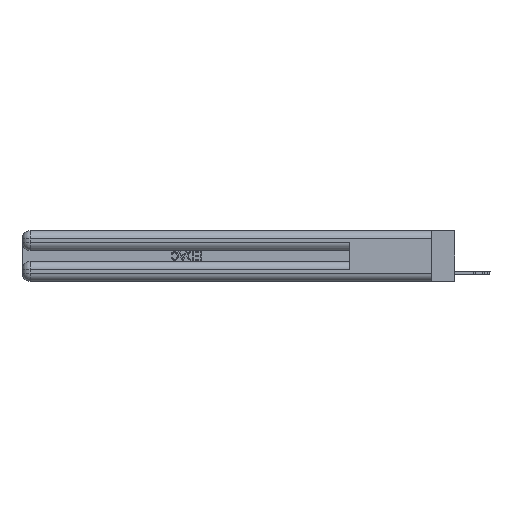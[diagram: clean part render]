
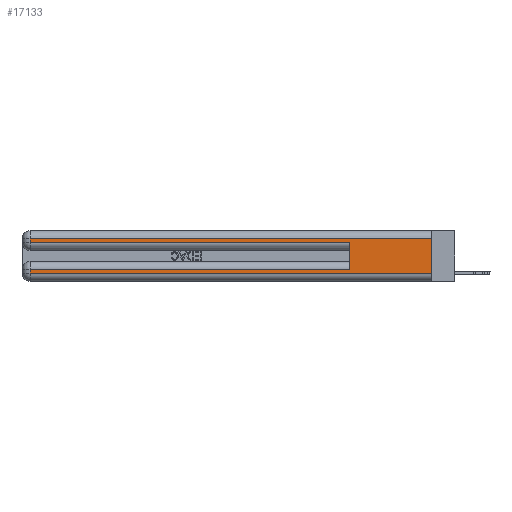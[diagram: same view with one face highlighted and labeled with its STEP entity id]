
A CAD part, left-side view. The second image highlights one B-rep face of the part: STEP entity #17133.
In plain terms, the highlighted planar face has unit normal (-1, 0, 0).
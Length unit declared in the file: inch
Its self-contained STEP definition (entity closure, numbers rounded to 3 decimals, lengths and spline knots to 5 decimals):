
#374 = CARTESIAN_POINT ( 'NONE',  ( 0., 0., 0.06 ) ) ;
#433 = FACE_OUTER_BOUND ( 'NONE', #507, .T. ) ;
#507 = EDGE_LOOP ( 'NONE', ( #16953, #8252, #4697, #8390, #25153, #7396, #28395, #18704 ) ) ;
#677 = CARTESIAN_POINT ( 'NONE',  ( 0., 0., 0.31 ) ) ;
#894 = DIRECTION ( 'NONE',  ( 0., 0., -1. ) ) ;
#1108 = EDGE_CURVE ( 'NONE', #17959, #3037, #18055, .T. ) ;
#1510 = VECTOR ( 'NONE', #14102, 39.37008 ) ;
#1527 = LINE ( 'NONE', #23000, #11461 ) ;
#2917 = CARTESIAN_POINT ( 'NONE',  ( 0., 0., 0.37 ) ) ;
#3037 = VERTEX_POINT ( 'NONE', #20757 ) ;
#3521 = CARTESIAN_POINT ( 'NONE',  ( 0., 2.94, 0.37 ) ) ;
#3586 = CARTESIAN_POINT ( 'NONE',  ( 0., 2.94, 0.06 ) ) ;
#4153 = VERTEX_POINT ( 'NONE', #19147 ) ;
#4234 = CARTESIAN_POINT ( 'NONE',  ( 0., 0., 0.31 ) ) ;
#4697 = ORIENTED_EDGE ( 'NONE', *, *, #22852, .T. ) ;
#5137 = DIRECTION ( 'NONE',  ( 1., 0., 0. ) ) ;
#6233 = DIRECTION ( 'NONE',  ( 0., 0., -1. ) ) ;
#6943 = LINE ( 'NONE', #16425, #1510 ) ;
#6964 = VERTEX_POINT ( 'NONE', #7858 ) ;
#7396 = ORIENTED_EDGE ( 'NONE', *, *, #19251, .T. ) ;
#7858 = CARTESIAN_POINT ( 'NONE',  ( 0., 2.94, 0.085 ) ) ;
#7879 = DIRECTION ( 'NONE',  ( 0., -1., 0. ) ) ;
#8252 = ORIENTED_EDGE ( 'NONE', *, *, #15559, .T. ) ;
#8390 = ORIENTED_EDGE ( 'NONE', *, *, #8533, .T. ) ;
#8533 = EDGE_CURVE ( 'NONE', #4153, #27915, #6943, .T. ) ;
#9976 = VECTOR ( 'NONE', #13878, 39.37008 ) ;
#11461 = VECTOR ( 'NONE', #22686, 39.37008 ) ;
#12382 = LINE ( 'NONE', #374, #20361 ) ;
#13648 = VECTOR ( 'NONE', #894, 39.37008 ) ;
#13878 = DIRECTION ( 'NONE',  ( 0., 0., 1. ) ) ;
#14102 = DIRECTION ( 'NONE',  ( 0., -1., 0. ) ) ;
#14308 = PLANE ( 'NONE',  #22790 ) ;
#14816 = VECTOR ( 'NONE', #15002, 39.37008 ) ;
#14874 = EDGE_CURVE ( 'NONE', #26285, #3037, #12382, .T. ) ;
#15002 = DIRECTION ( 'NONE',  ( 0., 1., 0. ) ) ;
#15559 = EDGE_CURVE ( 'NONE', #17959, #17238, #15589, .T. ) ;
#15589 = LINE ( 'NONE', #4234, #27515 ) ;
#16214 = LINE ( 'NONE', #25696, #9976 ) ;
#16425 = CARTESIAN_POINT ( 'NONE',  ( 0., 0., 0.285 ) ) ;
#16583 = CARTESIAN_POINT ( 'NONE',  ( 0., 0.6, 0.085 ) ) ;
#16953 = ORIENTED_EDGE ( 'NONE', *, *, #1108, .F. ) ;
#17133 = ADVANCED_FACE ( 'NONE', ( #433 ), #14308, .F. ) ;
#17238 = VERTEX_POINT ( 'NONE', #18021 ) ;
#17959 = VERTEX_POINT ( 'NONE', #677 ) ;
#18021 = CARTESIAN_POINT ( 'NONE',  ( 0., 2.94, 0.31 ) ) ;
#18055 = LINE ( 'NONE', #27539, #25703 ) ;
#18704 = ORIENTED_EDGE ( 'NONE', *, *, #14874, .T. ) ;
#18816 = CARTESIAN_POINT ( 'NONE',  ( 0., 0.6, 0.285 ) ) ;
#19147 = CARTESIAN_POINT ( 'NONE',  ( 0., 2.94, 0.285 ) ) ;
#19251 = EDGE_CURVE ( 'NONE', #22092, #6964, #26828, .T. ) ;
#20361 = VECTOR ( 'NONE', #7879, 39.37008 ) ;
#20757 = CARTESIAN_POINT ( 'NONE',  ( 0., 0., 0.06 ) ) ;
#22092 = VERTEX_POINT ( 'NONE', #16583 ) ;
#22686 = DIRECTION ( 'NONE',  ( 0., 0., -1. ) ) ;
#22790 = AXIS2_PLACEMENT_3D ( 'NONE', #2917, #5137, #26747 ) ;
#22852 = EDGE_CURVE ( 'NONE', #17238, #4153, #1527, .T. ) ;
#23000 = CARTESIAN_POINT ( 'NONE',  ( 0., 2.94, 0.37 ) ) ;
#24233 = LINE ( 'NONE', #3521, #13648 ) ;
#24309 = EDGE_CURVE ( 'NONE', #22092, #27915, #16214, .T. ) ;
#25153 = ORIENTED_EDGE ( 'NONE', *, *, #24309, .F. ) ;
#25696 = CARTESIAN_POINT ( 'NONE',  ( 0., 0.6, 0.145 ) ) ;
#25703 = VECTOR ( 'NONE', #6233, 39.37008 ) ;
#26285 = VERTEX_POINT ( 'NONE', #3586 ) ;
#26747 = DIRECTION ( 'NONE',  ( 0., 0., -1. ) ) ;
#26828 = LINE ( 'NONE', #29463, #14816 ) ;
#27515 = VECTOR ( 'NONE', #30201, 39.37008 ) ;
#27539 = CARTESIAN_POINT ( 'NONE',  ( 0., 0., 0.37 ) ) ;
#27915 = VERTEX_POINT ( 'NONE', #18816 ) ;
#28395 = ORIENTED_EDGE ( 'NONE', *, *, #29456, .T. ) ;
#29456 = EDGE_CURVE ( 'NONE', #6964, #26285, #24233, .T. ) ;
#29463 = CARTESIAN_POINT ( 'NONE',  ( 0., 0., 0.085 ) ) ;
#30201 = DIRECTION ( 'NONE',  ( 0., 1., 0. ) ) ;
